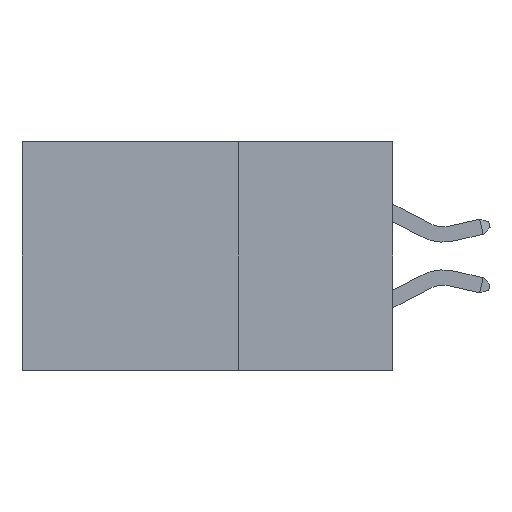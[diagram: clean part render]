
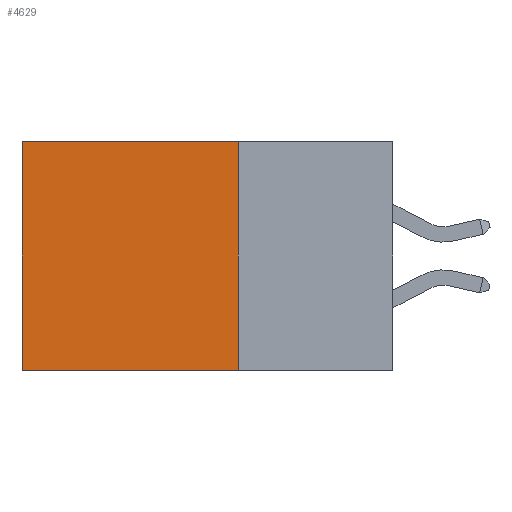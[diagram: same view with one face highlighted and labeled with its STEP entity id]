
A CAD part, left-side view. The second image highlights one B-rep face of the part: STEP entity #4629.
In plain terms, the highlighted planar face has unit normal (-1, 0, 0).
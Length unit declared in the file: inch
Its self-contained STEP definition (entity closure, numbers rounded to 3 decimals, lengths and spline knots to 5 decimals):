
#1507 = DIRECTION ( 'NONE',  ( 0., 0., -1. ) ) ;
#1723 = CARTESIAN_POINT ( 'NONE',  ( 0.2875, 0.25, 0. ) ) ;
#2417 = VECTOR ( 'NONE', #19891, 39.37008 ) ;
#2431 = ORIENTED_EDGE ( 'NONE', *, *, #5934, .T. ) ;
#2494 = LINE ( 'NONE', #9078, #18184 ) ;
#2522 = CARTESIAN_POINT ( 'NONE',  ( 0.2875, 0.6, 0. ) ) ;
#3298 = ORIENTED_EDGE ( 'NONE', *, *, #17038, .F. ) ;
#3725 = VECTOR ( 'NONE', #1507, 39.37008 ) ;
#4629 = ADVANCED_FACE ( 'NONE', ( #13107 ), #16081, .F. ) ;
#5507 = LINE ( 'NONE', #1723, #2417 ) ;
#5806 = VERTEX_POINT ( 'NONE', #20244 ) ;
#5934 = EDGE_CURVE ( 'NONE', #5806, #14359, #2494, .T. ) ;
#6034 = VERTEX_POINT ( 'NONE', #16439 ) ;
#6792 = EDGE_LOOP ( 'NONE', ( #14603, #16292, #3298, #2431 ) ) ;
#6950 = VECTOR ( 'NONE', #18967, 39.37008 ) ;
#8054 = CARTESIAN_POINT ( 'NONE',  ( 0.2875, 0.25, 0. ) ) ;
#8109 = CARTESIAN_POINT ( 'NONE',  ( 0.2875, 0.25, -0.37 ) ) ;
#8386 = CARTESIAN_POINT ( 'NONE',  ( 0.2875, 0.6, 0. ) ) ;
#9078 = CARTESIAN_POINT ( 'NONE',  ( 0.2875, 0.25, 0. ) ) ;
#9273 = DIRECTION ( 'NONE',  ( 0., 1., 0. ) ) ;
#9654 = DIRECTION ( 'NONE',  ( 0., 0., -1. ) ) ;
#9767 = DIRECTION ( 'NONE',  ( 1., 0., 0. ) ) ;
#11215 = VERTEX_POINT ( 'NONE', #8109 ) ;
#12394 = CARTESIAN_POINT ( 'NONE',  ( 0.2875, 0.25, -0.37 ) ) ;
#13107 = FACE_OUTER_BOUND ( 'NONE', #6792, .T. ) ;
#14359 = VERTEX_POINT ( 'NONE', #8386 ) ;
#14603 = ORIENTED_EDGE ( 'NONE', *, *, #18096, .T. ) ;
#15490 = EDGE_CURVE ( 'NONE', #11215, #6034, #18634, .T. ) ;
#16081 = PLANE ( 'NONE',  #19574 ) ;
#16237 = LINE ( 'NONE', #2522, #3725 ) ;
#16292 = ORIENTED_EDGE ( 'NONE', *, *, #15490, .F. ) ;
#16439 = CARTESIAN_POINT ( 'NONE',  ( 0.2875, 0.6, -0.37 ) ) ;
#17038 = EDGE_CURVE ( 'NONE', #5806, #11215, #5507, .T. ) ;
#18096 = EDGE_CURVE ( 'NONE', #14359, #6034, #16237, .T. ) ;
#18184 = VECTOR ( 'NONE', #9273, 39.37008 ) ;
#18634 = LINE ( 'NONE', #12394, #6950 ) ;
#18967 = DIRECTION ( 'NONE',  ( 0., 1., 0. ) ) ;
#19574 = AXIS2_PLACEMENT_3D ( 'NONE', #8054, #9767, #9654 ) ;
#19891 = DIRECTION ( 'NONE',  ( 0., 0., -1. ) ) ;
#20244 = CARTESIAN_POINT ( 'NONE',  ( 0.2875, 0.25, 0. ) ) ;
